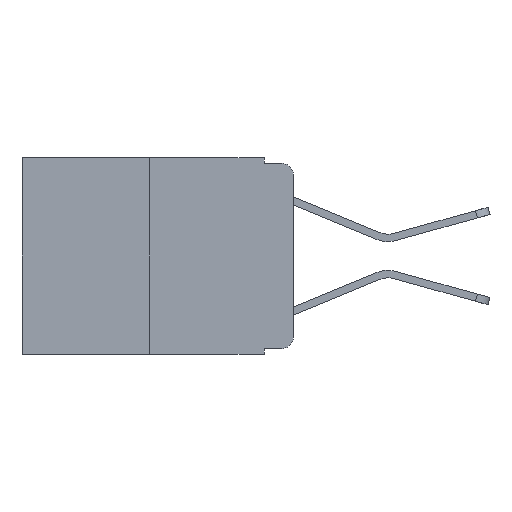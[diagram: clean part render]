
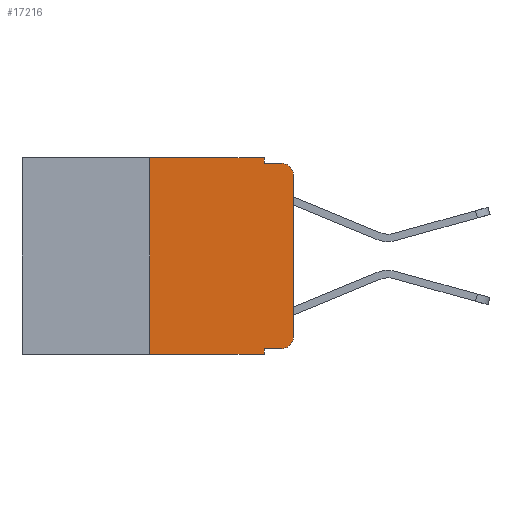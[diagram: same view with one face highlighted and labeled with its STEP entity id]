
A CAD part, left-side view. The second image highlights one B-rep face of the part: STEP entity #17216.
In plain terms, the highlighted planar face has unit normal (-1, 0, 0).
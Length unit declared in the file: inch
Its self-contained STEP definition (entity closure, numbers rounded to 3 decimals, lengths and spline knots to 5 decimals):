
#64 = VECTOR ( 'NONE', #10356, 39.37008 ) ;
#175 = CARTESIAN_POINT ( 'NONE',  ( 0., 0.051, -0.01 ) ) ;
#403 = AXIS2_PLACEMENT_3D ( 'NONE', #5223, #16416, #6839 ) ;
#434 = LINE ( 'NONE', #175, #12921 ) ;
#571 = EDGE_CURVE ( 'NONE', #1445, #19954, #16136, .T. ) ;
#804 = AXIS2_PLACEMENT_3D ( 'NONE', #2137, #13450, #3797 ) ;
#1176 = EDGE_CURVE ( 'NONE', #13350, #12729, #9884, .T. ) ;
#1332 = VERTEX_POINT ( 'NONE', #6901 ) ;
#1445 = VERTEX_POINT ( 'NONE', #7949 ) ;
#1498 = ORIENTED_EDGE ( 'NONE', *, *, #20560, .T. ) ;
#1615 = CARTESIAN_POINT ( 'NONE',  ( 0., 0.051, -0.333 ) ) ;
#1616 = CARTESIAN_POINT ( 'NONE',  ( 0., 0.051, 0. ) ) ;
#1731 = ORIENTED_EDGE ( 'NONE', *, *, #571, .T. ) ;
#1746 = VECTOR ( 'NONE', #5074, 39.37008 ) ;
#1882 = DIRECTION ( 'NONE',  ( 0., 0., -1. ) ) ;
#1981 = CARTESIAN_POINT ( 'NONE',  ( 0., 0.051, 0. ) ) ;
#2137 = CARTESIAN_POINT ( 'NONE',  ( 0., 0.473, 0. ) ) ;
#2324 = CARTESIAN_POINT ( 'NONE',  ( 0., 0., 0. ) ) ;
#2580 = ORIENTED_EDGE ( 'NONE', *, *, #5160, .F. ) ;
#2707 = AXIS2_PLACEMENT_3D ( 'NONE', #16294, #8993, #18735 ) ;
#2735 = ORIENTED_EDGE ( 'NONE', *, *, #3929, .F. ) ;
#2850 = EDGE_CURVE ( 'NONE', #15729, #13350, #18265, .T. ) ;
#2872 = ORIENTED_EDGE ( 'NONE', *, *, #1176, .F. ) ;
#3752 = ORIENTED_EDGE ( 'NONE', *, *, #2850, .F. ) ;
#3797 = DIRECTION ( 'NONE',  ( 0., 0., -1. ) ) ;
#3929 = EDGE_CURVE ( 'NONE', #12729, #14024, #10954, .T. ) ;
#3942 = CARTESIAN_POINT ( 'NONE',  ( 0., 0.25, 0. ) ) ;
#3977 = EDGE_LOOP ( 'NONE', ( #1498, #1731, #2580, #2735, #2872, #3752, #4705, #4822, #8805, #11572 ) ) ;
#4705 = ORIENTED_EDGE ( 'NONE', *, *, #9328, .T. ) ;
#4822 = ORIENTED_EDGE ( 'NONE', *, *, #14703, .F. ) ;
#5074 = DIRECTION ( 'NONE',  ( 0., -1., 0. ) ) ;
#5160 = EDGE_CURVE ( 'NONE', #14024, #19954, #434, .T. ) ;
#5223 = CARTESIAN_POINT ( 'NONE',  ( 0., 0.02, -0.313 ) ) ;
#6665 = LINE ( 'NONE', #7207, #7149 ) ;
#6839 = DIRECTION ( 'NONE',  ( 0., 0., -1. ) ) ;
#6901 = CARTESIAN_POINT ( 'NONE',  ( 0., 0.051, -0.343 ) ) ;
#7149 = VECTOR ( 'NONE', #18400, 39.37008 ) ;
#7198 = VECTOR ( 'NONE', #1882, 39.37008 ) ;
#7207 = CARTESIAN_POINT ( 'NONE',  ( 0., 0.051, -0.333 ) ) ;
#7865 = CARTESIAN_POINT ( 'NONE',  ( 0., 0.25, -0.343 ) ) ;
#7949 = CARTESIAN_POINT ( 'NONE',  ( 0., 0., -0.03 ) ) ;
#7970 = VECTOR ( 'NONE', #12029, 39.37008 ) ;
#8225 = FACE_OUTER_BOUND ( 'NONE', #3977, .T. ) ;
#8431 = CARTESIAN_POINT ( 'NONE',  ( 0., 0.051, 0. ) ) ;
#8756 = CARTESIAN_POINT ( 'NONE',  ( 0., 0.473, -0.343 ) ) ;
#8805 = ORIENTED_EDGE ( 'NONE', *, *, #13651, .T. ) ;
#8993 = DIRECTION ( 'NONE',  ( -1., 0., 0. ) ) ;
#9328 = EDGE_CURVE ( 'NONE', #15729, #1332, #13092, .T. ) ;
#9884 = LINE ( 'NONE', #12228, #1746 ) ;
#10257 = VECTOR ( 'NONE', #19932, 39.37008 ) ;
#10356 = DIRECTION ( 'NONE',  ( 0., -1., 0. ) ) ;
#10954 = LINE ( 'NONE', #8431, #7198 ) ;
#11214 = CARTESIAN_POINT ( 'NONE',  ( 0., 0.25, 0. ) ) ;
#11320 = CARTESIAN_POINT ( 'NONE',  ( 0., 0.02, -0.01 ) ) ;
#11572 = ORIENTED_EDGE ( 'NONE', *, *, #20060, .T. ) ;
#11674 = DIRECTION ( 'NONE',  ( 0., 0., -1. ) ) ;
#11884 = CIRCLE ( 'NONE', #403, 0.02 ) ;
#12029 = DIRECTION ( 'NONE',  ( 0., 0., 1. ) ) ;
#12228 = CARTESIAN_POINT ( 'NONE',  ( 0., 0.473, 0. ) ) ;
#12729 = VERTEX_POINT ( 'NONE', #1616 ) ;
#12740 = CARTESIAN_POINT ( 'NONE',  ( 0., 0., -0.313 ) ) ;
#12820 = CARTESIAN_POINT ( 'NONE',  ( 0., 0.02, -0.333 ) ) ;
#12921 = VECTOR ( 'NONE', #14811, 39.37008 ) ;
#13092 = LINE ( 'NONE', #8756, #64 ) ;
#13350 = VERTEX_POINT ( 'NONE', #11214 ) ;
#13450 = DIRECTION ( 'NONE',  ( 1., 0., 0. ) ) ;
#13651 = EDGE_CURVE ( 'NONE', #18216, #17528, #6665, .T. ) ;
#13849 = LINE ( 'NONE', #1981, #17595 ) ;
#14024 = VERTEX_POINT ( 'NONE', #14757 ) ;
#14609 = VERTEX_POINT ( 'NONE', #12740 ) ;
#14703 = EDGE_CURVE ( 'NONE', #18216, #1332, #13849, .T. ) ;
#14757 = CARTESIAN_POINT ( 'NONE',  ( 0., 0.051, -0.01 ) ) ;
#14811 = DIRECTION ( 'NONE',  ( 0., -1., 0. ) ) ;
#14970 = PLANE ( 'NONE',  #804 ) ;
#15729 = VERTEX_POINT ( 'NONE', #7865 ) ;
#16136 = CIRCLE ( 'NONE', #2707, 0.02 ) ;
#16294 = CARTESIAN_POINT ( 'NONE',  ( 0., 0.02, -0.03 ) ) ;
#16416 = DIRECTION ( 'NONE',  ( -1., 0., 0. ) ) ;
#16963 = LINE ( 'NONE', #2324, #7970 ) ;
#17216 = ADVANCED_FACE ( 'NONE', ( #8225 ), #14970, .F. ) ;
#17528 = VERTEX_POINT ( 'NONE', #12820 ) ;
#17595 = VECTOR ( 'NONE', #11674, 39.37008 ) ;
#18216 = VERTEX_POINT ( 'NONE', #1615 ) ;
#18265 = LINE ( 'NONE', #3942, #10257 ) ;
#18400 = DIRECTION ( 'NONE',  ( 0., -1., 0. ) ) ;
#18735 = DIRECTION ( 'NONE',  ( 0., 0., -1. ) ) ;
#19932 = DIRECTION ( 'NONE',  ( 0., 0., 1. ) ) ;
#19954 = VERTEX_POINT ( 'NONE', #11320 ) ;
#20060 = EDGE_CURVE ( 'NONE', #17528, #14609, #11884, .T. ) ;
#20560 = EDGE_CURVE ( 'NONE', #14609, #1445, #16963, .T. ) ;
